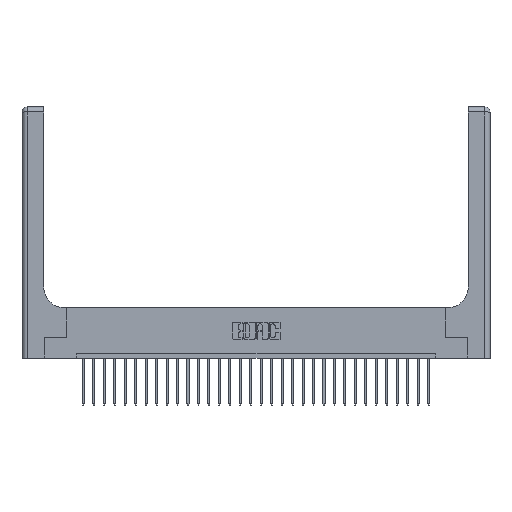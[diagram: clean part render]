
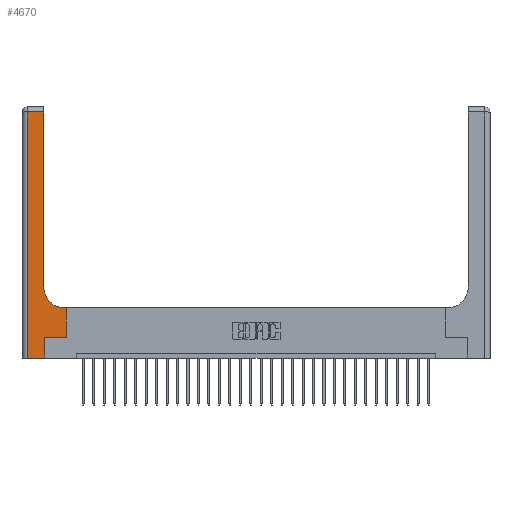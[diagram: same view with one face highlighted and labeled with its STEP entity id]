
A CAD part, top view. The second image highlights one B-rep face of the part: STEP entity #4670.
In plain terms, the highlighted planar face has unit normal (0, 0, 1).
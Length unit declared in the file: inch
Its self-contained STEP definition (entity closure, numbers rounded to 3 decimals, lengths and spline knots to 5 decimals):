
#137 = DIRECTION ( 'NONE',  ( -1., 0., 0. ) ) ;
#1419 = CARTESIAN_POINT ( 'NONE',  ( 0.51, 0.85, 0.37 ) ) ;
#1514 = CARTESIAN_POINT ( 'NONE',  ( 0.26, 3., 0.37 ) ) ;
#1734 = ORIENTED_EDGE ( 'NONE', *, *, #15259, .T. ) ;
#2106 = CARTESIAN_POINT ( 'NONE',  ( 0.265, 0.25, 0.37 ) ) ;
#2122 = ORIENTED_EDGE ( 'NONE', *, *, #17996, .T. ) ;
#2421 = EDGE_CURVE ( 'NONE', #26752, #12739, #14172, .T. ) ;
#2443 = ORIENTED_EDGE ( 'NONE', *, *, #16784, .T. ) ;
#2553 = EDGE_CURVE ( 'NONE', #15634, #5267, #20804, .T. ) ;
#2929 = DIRECTION ( 'NONE',  ( 0., -1., 0. ) ) ;
#3001 = VECTOR ( 'NONE', #14576, 39.37008 ) ;
#3188 = DIRECTION ( 'NONE',  ( 1., 0., 0. ) ) ;
#3894 = DIRECTION ( 'NONE',  ( -1., 0., 0. ) ) ;
#4270 = DIRECTION ( 'NONE',  ( 1., 0., 0. ) ) ;
#4670 = ADVANCED_FACE ( 'NONE', ( #6901 ), #11124, .F. ) ;
#5267 = VERTEX_POINT ( 'NONE', #21677 ) ;
#5384 = CARTESIAN_POINT ( 'NONE',  ( 0.265, 0., 0.37 ) ) ;
#5466 = CARTESIAN_POINT ( 'NONE',  ( 0.528, 0.6, 0.37 ) ) ;
#5482 = VECTOR ( 'NONE', #137, 39.37008 ) ;
#5616 = ORIENTED_EDGE ( 'NONE', *, *, #2553, .T. ) ;
#6478 = VECTOR ( 'NONE', #14343, 39.37008 ) ;
#6901 = FACE_OUTER_BOUND ( 'NONE', #7744, .T. ) ;
#7125 = ORIENTED_EDGE ( 'NONE', *, *, #2421, .T. ) ;
#7673 = VERTEX_POINT ( 'NONE', #25937 ) ;
#7744 = EDGE_LOOP ( 'NONE', ( #5616, #8777, #7125, #1734, #23850, #2443, #13943, #2122, #8530 ) ) ;
#7950 = VERTEX_POINT ( 'NONE', #23903 ) ;
#8530 = ORIENTED_EDGE ( 'NONE', *, *, #23569, .T. ) ;
#8777 = ORIENTED_EDGE ( 'NONE', *, *, #10386, .T. ) ;
#9019 = CARTESIAN_POINT ( 'NONE',  ( 0., 3., 0.37 ) ) ;
#10386 = EDGE_CURVE ( 'NONE', #5267, #26752, #16994, .T. ) ;
#10660 = DIRECTION ( 'NONE',  ( 0., 1., 0. ) ) ;
#11124 = PLANE ( 'NONE',  #25981 ) ;
#11916 = VERTEX_POINT ( 'NONE', #5466 ) ;
#12107 = CARTESIAN_POINT ( 'NONE',  ( 0.06, 0., 0.37 ) ) ;
#12739 = VERTEX_POINT ( 'NONE', #12107 ) ;
#12768 = CIRCLE ( 'NONE', #25373, 0.25 ) ;
#12905 = CARTESIAN_POINT ( 'NONE',  ( 0.528, 0.25, 0.37 ) ) ;
#13080 = VECTOR ( 'NONE', #3894, 39.37008 ) ;
#13943 = ORIENTED_EDGE ( 'NONE', *, *, #14507, .T. ) ;
#14172 = LINE ( 'NONE', #22231, #21907 ) ;
#14343 = DIRECTION ( 'NONE',  ( 0., 1., 0. ) ) ;
#14507 = EDGE_CURVE ( 'NONE', #7673, #11916, #16977, .T. ) ;
#14576 = DIRECTION ( 'NONE',  ( 0., 1., 0. ) ) ;
#15259 = EDGE_CURVE ( 'NONE', #12739, #17386, #26963, .T. ) ;
#15462 = DIRECTION ( 'NONE',  ( -1., 0., 0. ) ) ;
#15634 = VERTEX_POINT ( 'NONE', #20305 ) ;
#16784 = EDGE_CURVE ( 'NONE', #25986, #7673, #24881, .T. ) ;
#16793 = CARTESIAN_POINT ( 'NONE',  ( 0.06, 2.94, 0.37 ) ) ;
#16977 = LINE ( 'NONE', #12905, #20114 ) ;
#16994 = LINE ( 'NONE', #19409, #5482 ) ;
#17386 = VERTEX_POINT ( 'NONE', #5384 ) ;
#17996 = EDGE_CURVE ( 'NONE', #11916, #7950, #21347, .T. ) ;
#18297 = LINE ( 'NONE', #18717, #6478 ) ;
#18717 = CARTESIAN_POINT ( 'NONE',  ( 0.265, 0., 0.37 ) ) ;
#19409 = CARTESIAN_POINT ( 'NONE',  ( 0., 2.94, 0.37 ) ) ;
#20114 = VECTOR ( 'NONE', #10660, 39.37008 ) ;
#20296 = VECTOR ( 'NONE', #3188, 39.37008 ) ;
#20305 = CARTESIAN_POINT ( 'NONE',  ( 0.26, 0.85, 0.37 ) ) ;
#20804 = LINE ( 'NONE', #1514, #3001 ) ;
#21064 = VECTOR ( 'NONE', #4270, 39.37008 ) ;
#21347 = LINE ( 'NONE', #23195, #13080 ) ;
#21677 = CARTESIAN_POINT ( 'NONE',  ( 0.26, 2.94, 0.37 ) ) ;
#21907 = VECTOR ( 'NONE', #2929, 39.37008 ) ;
#22231 = CARTESIAN_POINT ( 'NONE',  ( 0.06, 3., 0.37 ) ) ;
#22769 = CARTESIAN_POINT ( 'NONE',  ( 0.265, 0.25, 0.37 ) ) ;
#23195 = CARTESIAN_POINT ( 'NONE',  ( 0.26, 0.6, 0.37 ) ) ;
#23435 = CARTESIAN_POINT ( 'NONE',  ( 0., 0., 0.37 ) ) ;
#23536 = EDGE_CURVE ( 'NONE', #17386, #25986, #18297, .T. ) ;
#23569 = EDGE_CURVE ( 'NONE', #7950, #15634, #12768, .T. ) ;
#23821 = DIRECTION ( 'NONE',  ( 0., 0., -1. ) ) ;
#23850 = ORIENTED_EDGE ( 'NONE', *, *, #23536, .T. ) ;
#23903 = CARTESIAN_POINT ( 'NONE',  ( 0.51, 0.6, 0.37 ) ) ;
#24660 = DIRECTION ( 'NONE',  ( 0., 0., -1. ) ) ;
#24881 = LINE ( 'NONE', #22769, #20296 ) ;
#25373 = AXIS2_PLACEMENT_3D ( 'NONE', #1419, #24660, #27050 ) ;
#25937 = CARTESIAN_POINT ( 'NONE',  ( 0.528, 0.25, 0.37 ) ) ;
#25981 = AXIS2_PLACEMENT_3D ( 'NONE', #9019, #23821, #15462 ) ;
#25986 = VERTEX_POINT ( 'NONE', #2106 ) ;
#26752 = VERTEX_POINT ( 'NONE', #16793 ) ;
#26963 = LINE ( 'NONE', #23435, #21064 ) ;
#27050 = DIRECTION ( 'NONE',  ( 1., 0., 0. ) ) ;
